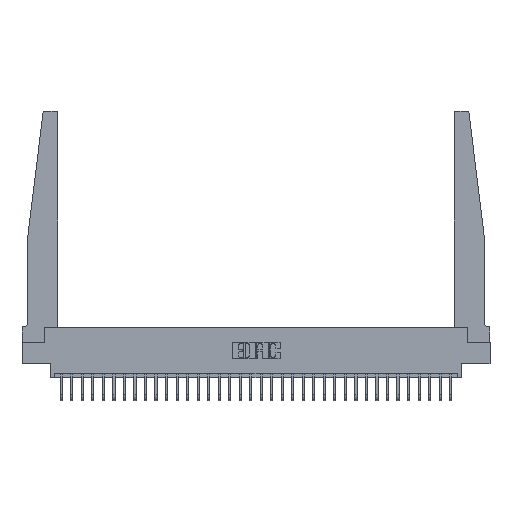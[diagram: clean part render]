
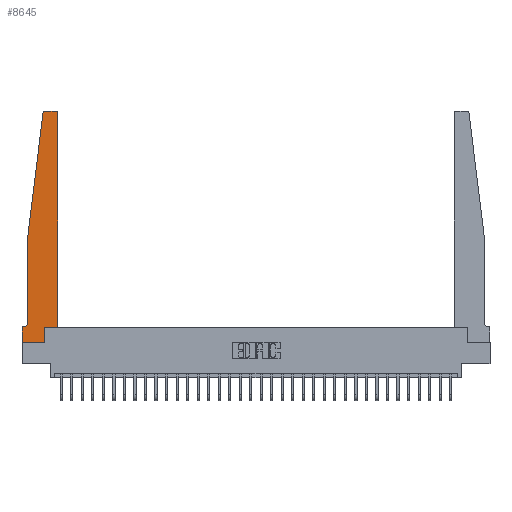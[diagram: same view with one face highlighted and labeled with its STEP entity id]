
A CAD part, top view. The second image highlights one B-rep face of the part: STEP entity #8645.
In plain terms, the highlighted planar face has unit normal (0, 0, 1).
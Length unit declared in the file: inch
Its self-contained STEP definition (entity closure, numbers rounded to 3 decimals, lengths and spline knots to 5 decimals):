
#234 = DIRECTION ( 'NONE',  ( -1., 0., 0. ) ) ;
#351 = VERTEX_POINT ( 'NONE', #21490 ) ;
#417 = LINE ( 'NONE', #9359, #2237 ) ;
#817 = LINE ( 'NONE', #2587, #15771 ) ;
#1836 = EDGE_CURVE ( 'NONE', #24930, #7675, #417, .T. ) ;
#2237 = VECTOR ( 'NONE', #11456, 39.37008 ) ;
#2587 = CARTESIAN_POINT ( 'NONE',  ( 0.065, 1.25, 0.37 ) ) ;
#3173 = EDGE_CURVE ( 'NONE', #23202, #3210, #817, .T. ) ;
#3210 = VERTEX_POINT ( 'NONE', #10051 ) ;
#3286 = CARTESIAN_POINT ( 'NONE',  ( 0.2605, 0.18, 0.37 ) ) ;
#3673 = EDGE_CURVE ( 'NONE', #20193, #351, #4313, .T. ) ;
#3882 = CARTESIAN_POINT ( 'NONE',  ( 0., 0., 0.37 ) ) ;
#4313 = LINE ( 'NONE', #3882, #14274 ) ;
#4386 = DIRECTION ( 'NONE',  ( 1., 0., 0. ) ) ;
#4479 = LINE ( 'NONE', #11495, #21209 ) ;
#4871 = LINE ( 'NONE', #25484, #5875 ) ;
#4911 = LINE ( 'NONE', #20581, #23128 ) ;
#5288 = ORIENTED_EDGE ( 'NONE', *, *, #9089, .T. ) ;
#5875 = VECTOR ( 'NONE', #16209, 39.37008 ) ;
#6470 = DIRECTION ( 'NONE',  ( 0., 0., 1. ) ) ;
#6731 = CIRCLE ( 'NONE', #13886, 0.05 ) ;
#7146 = ORIENTED_EDGE ( 'NONE', *, *, #11507, .T. ) ;
#7675 = VERTEX_POINT ( 'NONE', #19582 ) ;
#7779 = VECTOR ( 'NONE', #27956, 39.37008 ) ;
#8250 = ORIENTED_EDGE ( 'NONE', *, *, #3673, .T. ) ;
#8375 = DIRECTION ( 'NONE',  ( 0., 0., -1. ) ) ;
#8415 = FACE_OUTER_BOUND ( 'NONE', #14744, .T. ) ;
#8566 = PLANE ( 'NONE',  #23892 ) ;
#8645 = ADVANCED_FACE ( 'NONE', ( #8415 ), #8566, .T. ) ;
#9089 = EDGE_CURVE ( 'NONE', #11935, #28202, #6731, .T. ) ;
#9226 = DIRECTION ( 'NONE',  ( -1., 0., 0. ) ) ;
#9359 = CARTESIAN_POINT ( 'NONE',  ( 0.425, 0.18, 0.37 ) ) ;
#9463 = ORIENTED_EDGE ( 'NONE', *, *, #15050, .T. ) ;
#9672 = DIRECTION ( 'NONE',  ( 1., 0., 0. ) ) ;
#9824 = ORIENTED_EDGE ( 'NONE', *, *, #3173, .T. ) ;
#9905 = DIRECTION ( 'NONE',  ( -0.122, -0.992, 0. ) ) ;
#9941 = CIRCLE ( 'NONE', #26671, 0.03 ) ;
#10051 = CARTESIAN_POINT ( 'NONE',  ( 0.065, 1.25, 0.37 ) ) ;
#10148 = LINE ( 'NONE', #3286, #7779 ) ;
#10514 = CARTESIAN_POINT ( 'NONE',  ( 0.015, 0.1875, 0.37 ) ) ;
#11241 = DIRECTION ( 'NONE',  ( 1., 0., 0. ) ) ;
#11456 = DIRECTION ( 'NONE',  ( 0., 1., 0. ) ) ;
#11495 = CARTESIAN_POINT ( 'NONE',  ( 0., 0., 0.37 ) ) ;
#11507 = EDGE_CURVE ( 'NONE', #17352, #14973, #10148, .T. ) ;
#11564 = CARTESIAN_POINT ( 'NONE',  ( 0., 0.1875, 0.37 ) ) ;
#11915 = VECTOR ( 'NONE', #9672, 39.37008 ) ;
#11935 = VERTEX_POINT ( 'NONE', #12603 ) ;
#12603 = CARTESIAN_POINT ( 'NONE',  ( 0.065, 0.2375, 0.37 ) ) ;
#12624 = ORIENTED_EDGE ( 'NONE', *, *, #29417, .T. ) ;
#13465 = EDGE_CURVE ( 'NONE', #3210, #11935, #4871, .T. ) ;
#13730 = CARTESIAN_POINT ( 'NONE',  ( 0.2605, 0.18, 0.37 ) ) ;
#13886 = AXIS2_PLACEMENT_3D ( 'NONE', #26625, #8375, #24665 ) ;
#14274 = VECTOR ( 'NONE', #28988, 39.37008 ) ;
#14723 = ORIENTED_EDGE ( 'NONE', *, *, #22233, .T. ) ;
#14727 = VECTOR ( 'NONE', #234, 39.37008 ) ;
#14744 = EDGE_LOOP ( 'NONE', ( #14723, #19397, #9824, #29226, #5288, #16462, #8250, #9463, #7146, #12624, #22429, #26775 ) ) ;
#14973 = VERTEX_POINT ( 'NONE', #13730 ) ;
#15050 = EDGE_CURVE ( 'NONE', #351, #17352, #4479, .T. ) ;
#15771 = VECTOR ( 'NONE', #9905, 39.37008 ) ;
#16209 = DIRECTION ( 'NONE',  ( 0., -1., 0. ) ) ;
#16462 = ORIENTED_EDGE ( 'NONE', *, *, #26682, .T. ) ;
#17352 = VERTEX_POINT ( 'NONE', #22463 ) ;
#18778 = LINE ( 'NONE', #25076, #11915 ) ;
#19397 = ORIENTED_EDGE ( 'NONE', *, *, #25958, .T. ) ;
#19582 = CARTESIAN_POINT ( 'NONE',  ( 0.425, 2.72, 0.37 ) ) ;
#19984 = DIRECTION ( 'NONE',  ( 0., 0., 1. ) ) ;
#20193 = VERTEX_POINT ( 'NONE', #11564 ) ;
#20581 = CARTESIAN_POINT ( 'NONE',  ( 0.25, 2.75, 0.37 ) ) ;
#20602 = DIRECTION ( 'NONE',  ( 1., 0., 0. ) ) ;
#21001 = VERTEX_POINT ( 'NONE', #29086 ) ;
#21209 = VECTOR ( 'NONE', #20602, 39.37008 ) ;
#21357 = CARTESIAN_POINT ( 'NONE',  ( 0.395, 2.75, 0.37 ) ) ;
#21490 = CARTESIAN_POINT ( 'NONE',  ( 0., 0., 0.37 ) ) ;
#21869 = AXIS2_PLACEMENT_3D ( 'NONE', #26585, #19984, #24187 ) ;
#22233 = EDGE_CURVE ( 'NONE', #25889, #21001, #4911, .T. ) ;
#22398 = CARTESIAN_POINT ( 'NONE',  ( 0.425, 0.18, 0.37 ) ) ;
#22429 = ORIENTED_EDGE ( 'NONE', *, *, #1836, .T. ) ;
#22463 = CARTESIAN_POINT ( 'NONE',  ( 0.2605, 0., 0.37 ) ) ;
#23128 = VECTOR ( 'NONE', #9226, 39.37008 ) ;
#23202 = VERTEX_POINT ( 'NONE', #28876 ) ;
#23892 = AXIS2_PLACEMENT_3D ( 'NONE', #27252, #6470, #11241 ) ;
#24187 = DIRECTION ( 'NONE',  ( 1., 0., 0. ) ) ;
#24266 = CIRCLE ( 'NONE', #21869, 0.03 ) ;
#24665 = DIRECTION ( 'NONE',  ( -1., 0., 0. ) ) ;
#24860 = DIRECTION ( 'NONE',  ( 0., 0., 1. ) ) ;
#24930 = VERTEX_POINT ( 'NONE', #22398 ) ;
#25076 = CARTESIAN_POINT ( 'NONE',  ( 0.425, 0.18, 0.37 ) ) ;
#25477 = LINE ( 'NONE', #27584, #14727 ) ;
#25484 = CARTESIAN_POINT ( 'NONE',  ( 0.065, 1.25, 0.37 ) ) ;
#25889 = VERTEX_POINT ( 'NONE', #21357 ) ;
#25958 = EDGE_CURVE ( 'NONE', #21001, #23202, #24266, .T. ) ;
#26585 = CARTESIAN_POINT ( 'NONE',  ( 0.27653, 2.72, 0.37 ) ) ;
#26625 = CARTESIAN_POINT ( 'NONE',  ( 0.015, 0.2375, 0.37 ) ) ;
#26671 = AXIS2_PLACEMENT_3D ( 'NONE', #29207, #24860, #4386 ) ;
#26682 = EDGE_CURVE ( 'NONE', #28202, #20193, #25477, .T. ) ;
#26775 = ORIENTED_EDGE ( 'NONE', *, *, #28341, .T. ) ;
#27252 = CARTESIAN_POINT ( 'NONE',  ( 0., 0.1875, 0.37 ) ) ;
#27584 = CARTESIAN_POINT ( 'NONE',  ( 0.065, 0.1875, 0.37 ) ) ;
#27956 = DIRECTION ( 'NONE',  ( 0., 1., 0. ) ) ;
#28202 = VERTEX_POINT ( 'NONE', #10514 ) ;
#28341 = EDGE_CURVE ( 'NONE', #7675, #25889, #9941, .T. ) ;
#28876 = CARTESIAN_POINT ( 'NONE',  ( 0.24675, 2.72367, 0.37 ) ) ;
#28988 = DIRECTION ( 'NONE',  ( 0., -1., 0. ) ) ;
#29086 = CARTESIAN_POINT ( 'NONE',  ( 0.27653, 2.75, 0.37 ) ) ;
#29207 = CARTESIAN_POINT ( 'NONE',  ( 0.395, 2.72, 0.37 ) ) ;
#29226 = ORIENTED_EDGE ( 'NONE', *, *, #13465, .T. ) ;
#29417 = EDGE_CURVE ( 'NONE', #14973, #24930, #18778, .T. ) ;
